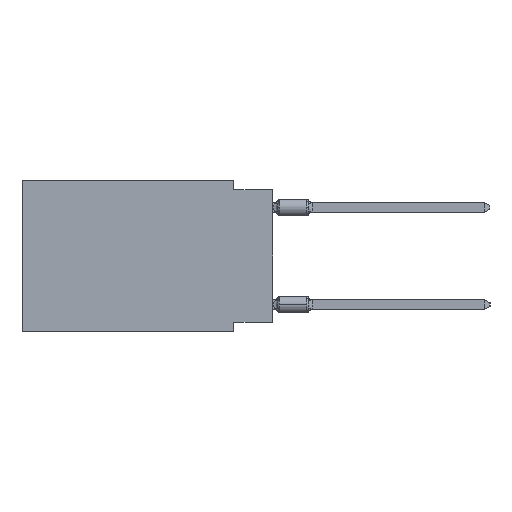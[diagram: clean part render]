
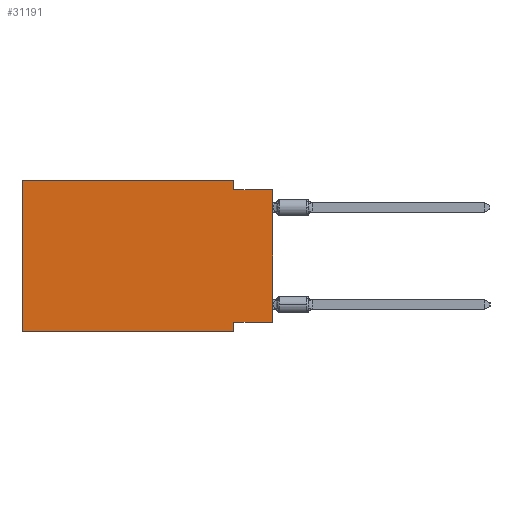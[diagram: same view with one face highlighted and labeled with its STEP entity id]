
A CAD part, left-side view. The second image highlights one B-rep face of the part: STEP entity #31191.
In plain terms, the highlighted planar face has unit normal (-1, 0, 0).
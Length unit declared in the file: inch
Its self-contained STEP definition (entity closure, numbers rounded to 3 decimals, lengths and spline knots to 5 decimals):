
#284 = DIRECTION ( 'NONE',  ( 1., 0., 0. ) ) ;
#534 = LINE ( 'NONE', #34748, #27568 ) ;
#632 = VECTOR ( 'NONE', #30970, 39.37008 ) ;
#734 = DIRECTION ( 'NONE',  ( 0., 0., -1. ) ) ;
#2737 = ORIENTED_EDGE ( 'NONE', *, *, #37032, .F. ) ;
#3662 = ORIENTED_EDGE ( 'NONE', *, *, #19682, .F. ) ;
#4105 = VERTEX_POINT ( 'NONE', #32127 ) ;
#4428 = VERTEX_POINT ( 'NONE', #16117 ) ;
#4958 = CARTESIAN_POINT ( 'NONE',  ( 0., 0.645, -0.39 ) ) ;
#6176 = ORIENTED_EDGE ( 'NONE', *, *, #33719, .T. ) ;
#6207 = CARTESIAN_POINT ( 'NONE',  ( 0., 0.645, 0. ) ) ;
#6735 = CARTESIAN_POINT ( 'NONE',  ( 0., 0., 0. ) ) ;
#6917 = VECTOR ( 'NONE', #22751, 39.37008 ) ;
#7912 = CARTESIAN_POINT ( 'NONE',  ( 0., 0., -0.365 ) ) ;
#8747 = VERTEX_POINT ( 'NONE', #31264 ) ;
#10178 = DIRECTION ( 'NONE',  ( 0., -1., 0. ) ) ;
#10978 = VECTOR ( 'NONE', #10178, 39.37008 ) ;
#11583 = CARTESIAN_POINT ( 'NONE',  ( 0., 0.1, -0.365 ) ) ;
#12307 = CARTESIAN_POINT ( 'NONE',  ( 0., 0.645, 0. ) ) ;
#12559 = ORIENTED_EDGE ( 'NONE', *, *, #32097, .T. ) ;
#14071 = VECTOR ( 'NONE', #31566, 39.37008 ) ;
#14208 = ORIENTED_EDGE ( 'NONE', *, *, #18162, .F. ) ;
#14374 = VERTEX_POINT ( 'NONE', #6207 ) ;
#14588 = VERTEX_POINT ( 'NONE', #11583 ) ;
#15383 = LINE ( 'NONE', #18781, #632 ) ;
#16117 = CARTESIAN_POINT ( 'NONE',  ( 0., 0.1, 0. ) ) ;
#16232 = DIRECTION ( 'NONE',  ( 0., 0., -1. ) ) ;
#16379 = LINE ( 'NONE', #6735, #14071 ) ;
#16675 = ORIENTED_EDGE ( 'NONE', *, *, #17095, .F. ) ;
#17095 = EDGE_CURVE ( 'NONE', #36871, #14588, #35331, .T. ) ;
#18042 = AXIS2_PLACEMENT_3D ( 'NONE', #12307, #284, #24535 ) ;
#18127 = CARTESIAN_POINT ( 'NONE',  ( 0., 0.1, -0.025 ) ) ;
#18162 = EDGE_CURVE ( 'NONE', #14588, #8747, #534, .T. ) ;
#18781 = CARTESIAN_POINT ( 'NONE',  ( 0., 0.645, 0. ) ) ;
#18910 = ORIENTED_EDGE ( 'NONE', *, *, #30823, .F. ) ;
#19398 = ORIENTED_EDGE ( 'NONE', *, *, #32955, .F. ) ;
#19470 = CARTESIAN_POINT ( 'NONE',  ( 0., 0., -0.365 ) ) ;
#19682 = EDGE_CURVE ( 'NONE', #4428, #34378, #26153, .T. ) ;
#20070 = CARTESIAN_POINT ( 'NONE',  ( 0., 0.645, 0. ) ) ;
#20274 = DIRECTION ( 'NONE',  ( 0., -1., 0. ) ) ;
#22304 = VERTEX_POINT ( 'NONE', #31210 ) ;
#22751 = DIRECTION ( 'NONE',  ( 0., 1., 0. ) ) ;
#22926 = EDGE_LOOP ( 'NONE', ( #12559, #2737, #3662, #19398, #18910, #6176, #14208, #16675 ) ) ;
#23851 = DIRECTION ( 'NONE',  ( 0., -1., 0. ) ) ;
#24335 = FACE_OUTER_BOUND ( 'NONE', #22926, .T. ) ;
#24535 = DIRECTION ( 'NONE',  ( 0., 0., -1. ) ) ;
#25014 = VECTOR ( 'NONE', #20274, 39.37008 ) ;
#25411 = LINE ( 'NONE', #4958, #10978 ) ;
#26153 = LINE ( 'NONE', #26355, #37880 ) ;
#26355 = CARTESIAN_POINT ( 'NONE',  ( 0., 0.1, 0. ) ) ;
#26839 = CARTESIAN_POINT ( 'NONE',  ( 0., 0., -0.025 ) ) ;
#27568 = VECTOR ( 'NONE', #734, 39.37008 ) ;
#27725 = PLANE ( 'NONE',  #18042 ) ;
#28313 = VECTOR ( 'NONE', #23851, 39.37008 ) ;
#29082 = LINE ( 'NONE', #20070, #25014 ) ;
#30823 = EDGE_CURVE ( 'NONE', #22304, #14374, #15383, .T. ) ;
#30970 = DIRECTION ( 'NONE',  ( 0., 0., 1. ) ) ;
#31191 = ADVANCED_FACE ( 'NONE', ( #24335 ), #27725, .F. ) ;
#31210 = CARTESIAN_POINT ( 'NONE',  ( 0., 0.645, -0.39 ) ) ;
#31264 = CARTESIAN_POINT ( 'NONE',  ( 0., 0.1, -0.39 ) ) ;
#31566 = DIRECTION ( 'NONE',  ( 0., 0., 1. ) ) ;
#32097 = EDGE_CURVE ( 'NONE', #36871, #4105, #16379, .T. ) ;
#32127 = CARTESIAN_POINT ( 'NONE',  ( 0., 0., -0.025 ) ) ;
#32955 = EDGE_CURVE ( 'NONE', #14374, #4428, #29082, .T. ) ;
#33719 = EDGE_CURVE ( 'NONE', #22304, #8747, #25411, .T. ) ;
#34378 = VERTEX_POINT ( 'NONE', #18127 ) ;
#34748 = CARTESIAN_POINT ( 'NONE',  ( 0., 0.1, -0.39 ) ) ;
#35331 = LINE ( 'NONE', #7912, #6917 ) ;
#36871 = VERTEX_POINT ( 'NONE', #19470 ) ;
#37032 = EDGE_CURVE ( 'NONE', #34378, #4105, #38666, .T. ) ;
#37880 = VECTOR ( 'NONE', #16232, 39.37008 ) ;
#38666 = LINE ( 'NONE', #26839, #28313 ) ;
